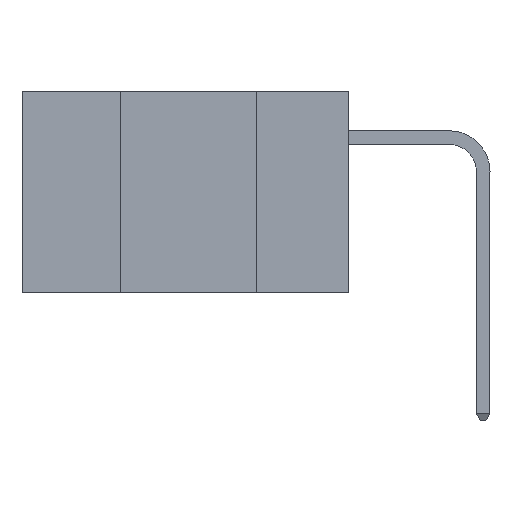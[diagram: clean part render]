
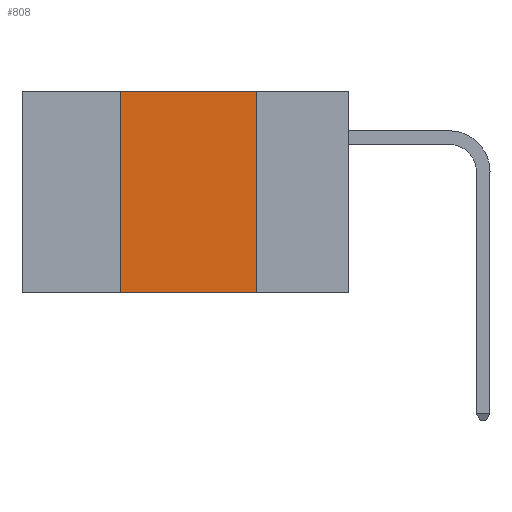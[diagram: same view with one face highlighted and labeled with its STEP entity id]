
A CAD part, left-side view. The second image highlights one B-rep face of the part: STEP entity #808.
In plain terms, the highlighted planar face has unit normal (-1, 0, 0).
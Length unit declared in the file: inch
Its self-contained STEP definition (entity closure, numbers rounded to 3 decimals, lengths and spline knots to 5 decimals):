
#363 = LINE ( 'NONE', #13663, #1135 ) ;
#477 = VECTOR ( 'NONE', #5615, 39.37008 ) ;
#808 = ADVANCED_FACE ( 'NONE', ( #14215 ), #6053, .F. ) ;
#1135 = VECTOR ( 'NONE', #11377, 39.37008 ) ;
#1220 = VERTEX_POINT ( 'NONE', #8529 ) ;
#1904 = CARTESIAN_POINT ( 'NONE',  ( 0., 0.6, 0. ) ) ;
#2606 = DIRECTION ( 'NONE',  ( 1., 0., 0. ) ) ;
#3100 = CARTESIAN_POINT ( 'NONE',  ( 0., 0.17, 0. ) ) ;
#3613 = LINE ( 'NONE', #3100, #477 ) ;
#3727 = CARTESIAN_POINT ( 'NONE',  ( 0., 0.6, 0. ) ) ;
#3841 = EDGE_CURVE ( 'NONE', #1220, #4872, #6145, .T. ) ;
#4620 = EDGE_LOOP ( 'NONE', ( #6116, #11520, #6578, #9791 ) ) ;
#4805 = DIRECTION ( 'NONE',  ( 0., 0., -1. ) ) ;
#4872 = VERTEX_POINT ( 'NONE', #7778 ) ;
#5104 = VERTEX_POINT ( 'NONE', #8354 ) ;
#5583 = EDGE_CURVE ( 'NONE', #5104, #7230, #363, .T. ) ;
#5615 = DIRECTION ( 'NONE',  ( 0., 0., -1. ) ) ;
#6053 = PLANE ( 'NONE',  #12795 ) ;
#6116 = ORIENTED_EDGE ( 'NONE', *, *, #7763, .F. ) ;
#6145 = LINE ( 'NONE', #1904, #8161 ) ;
#6578 = ORIENTED_EDGE ( 'NONE', *, *, #7741, .F. ) ;
#6768 = LINE ( 'NONE', #12295, #14041 ) ;
#7023 = CARTESIAN_POINT ( 'NONE',  ( 0., 0.17, -0.37 ) ) ;
#7230 = VERTEX_POINT ( 'NONE', #7023 ) ;
#7741 = EDGE_CURVE ( 'NONE', #5104, #1220, #6768, .T. ) ;
#7763 = EDGE_CURVE ( 'NONE', #4872, #7230, #3613, .T. ) ;
#7778 = CARTESIAN_POINT ( 'NONE',  ( 0., 0.17, 0. ) ) ;
#8161 = VECTOR ( 'NONE', #8957, 39.37008 ) ;
#8354 = CARTESIAN_POINT ( 'NONE',  ( 0., 0.42, -0.37 ) ) ;
#8529 = CARTESIAN_POINT ( 'NONE',  ( 0., 0.42, 0. ) ) ;
#8957 = DIRECTION ( 'NONE',  ( 0., -1., 0. ) ) ;
#9791 = ORIENTED_EDGE ( 'NONE', *, *, #5583, .T. ) ;
#11200 = DIRECTION ( 'NONE',  ( 0., 0., 1. ) ) ;
#11377 = DIRECTION ( 'NONE',  ( 0., -1., 0. ) ) ;
#11520 = ORIENTED_EDGE ( 'NONE', *, *, #3841, .F. ) ;
#12295 = CARTESIAN_POINT ( 'NONE',  ( 0., 0.42, 0. ) ) ;
#12795 = AXIS2_PLACEMENT_3D ( 'NONE', #3727, #2606, #4805 ) ;
#13663 = CARTESIAN_POINT ( 'NONE',  ( 0., 0.6, -0.37 ) ) ;
#14041 = VECTOR ( 'NONE', #11200, 39.37008 ) ;
#14215 = FACE_OUTER_BOUND ( 'NONE', #4620, .T. ) ;
